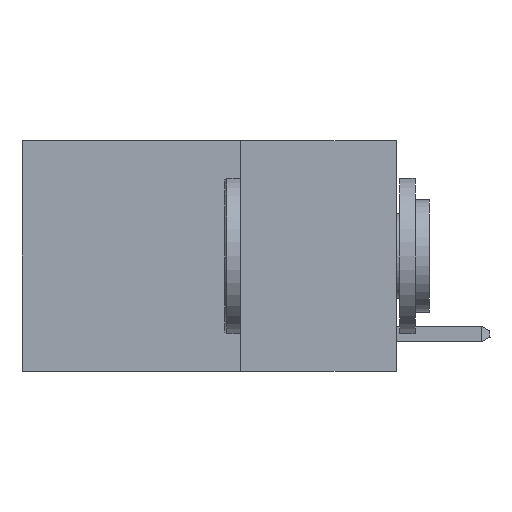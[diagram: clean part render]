
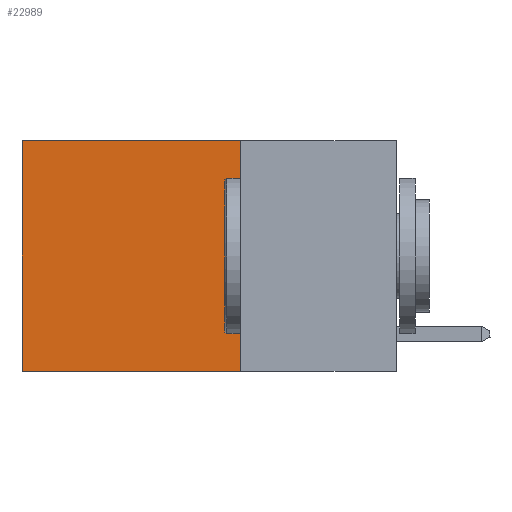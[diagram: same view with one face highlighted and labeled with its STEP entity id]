
A CAD part, left-side view. The second image highlights one B-rep face of the part: STEP entity #22989.
In plain terms, the highlighted planar face has unit normal (-1, 0, 0).
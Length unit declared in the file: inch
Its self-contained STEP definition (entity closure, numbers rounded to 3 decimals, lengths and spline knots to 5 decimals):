
#528 = ORIENTED_EDGE ( 'NONE', *, *, #19490, .F. ) ;
#569 = DIRECTION ( 'NONE',  ( 0., 0., -1. ) ) ;
#1579 = CARTESIAN_POINT ( 'NONE',  ( 0.2625, 0.25, 0. ) ) ;
#1910 = VECTOR ( 'NONE', #569, 39.37008 ) ;
#2609 = DIRECTION ( 'NONE',  ( 0., 1., 0. ) ) ;
#3586 = CARTESIAN_POINT ( 'NONE',  ( 0.2625, 0.25, 0. ) ) ;
#4742 = LINE ( 'NONE', #24631, #25064 ) ;
#5304 = EDGE_CURVE ( 'NONE', #22569, #21810, #12708, .T. ) ;
#6697 = VERTEX_POINT ( 'NONE', #18806 ) ;
#9290 = DIRECTION ( 'NONE',  ( 0., 1., 0. ) ) ;
#11792 = DIRECTION ( 'NONE',  ( 1., 0., 0. ) ) ;
#12708 = LINE ( 'NONE', #20767, #24083 ) ;
#13017 = CARTESIAN_POINT ( 'NONE',  ( 0.2625, 0.6, 0. ) ) ;
#14686 = ORIENTED_EDGE ( 'NONE', *, *, #15595, .T. ) ;
#15595 = EDGE_CURVE ( 'NONE', #18092, #6697, #23070, .T. ) ;
#15788 = EDGE_CURVE ( 'NONE', #22569, #18092, #21730, .T. ) ;
#16154 = FACE_OUTER_BOUND ( 'NONE', #24456, .T. ) ;
#18092 = VERTEX_POINT ( 'NONE', #18758 ) ;
#18519 = DIRECTION ( 'NONE',  ( 0., 0., -1. ) ) ;
#18758 = CARTESIAN_POINT ( 'NONE',  ( 0.2625, 0.6, 0. ) ) ;
#18792 = ORIENTED_EDGE ( 'NONE', *, *, #5304, .F. ) ;
#18806 = CARTESIAN_POINT ( 'NONE',  ( 0.2625, 0.6, -0.37 ) ) ;
#19490 = EDGE_CURVE ( 'NONE', #21810, #6697, #4742, .T. ) ;
#19782 = CARTESIAN_POINT ( 'NONE',  ( 0.2625, 0.25, 0. ) ) ;
#20099 = VECTOR ( 'NONE', #9290, 39.37008 ) ;
#20767 = CARTESIAN_POINT ( 'NONE',  ( 0.2625, 0.25, 0. ) ) ;
#20942 = AXIS2_PLACEMENT_3D ( 'NONE', #1579, #11792, #24238 ) ;
#21730 = LINE ( 'NONE', #3586, #20099 ) ;
#21810 = VERTEX_POINT ( 'NONE', #24501 ) ;
#22377 = PLANE ( 'NONE',  #20942 ) ;
#22569 = VERTEX_POINT ( 'NONE', #19782 ) ;
#22976 = ORIENTED_EDGE ( 'NONE', *, *, #15788, .T. ) ;
#22989 = ADVANCED_FACE ( 'NONE', ( #16154 ), #22377, .F. ) ;
#23070 = LINE ( 'NONE', #13017, #1910 ) ;
#24083 = VECTOR ( 'NONE', #18519, 39.37008 ) ;
#24238 = DIRECTION ( 'NONE',  ( 0., 0., -1. ) ) ;
#24456 = EDGE_LOOP ( 'NONE', ( #14686, #528, #18792, #22976 ) ) ;
#24501 = CARTESIAN_POINT ( 'NONE',  ( 0.2625, 0.25, -0.37 ) ) ;
#24631 = CARTESIAN_POINT ( 'NONE',  ( 0.2625, 0.25, -0.37 ) ) ;
#25064 = VECTOR ( 'NONE', #2609, 39.37008 ) ;
